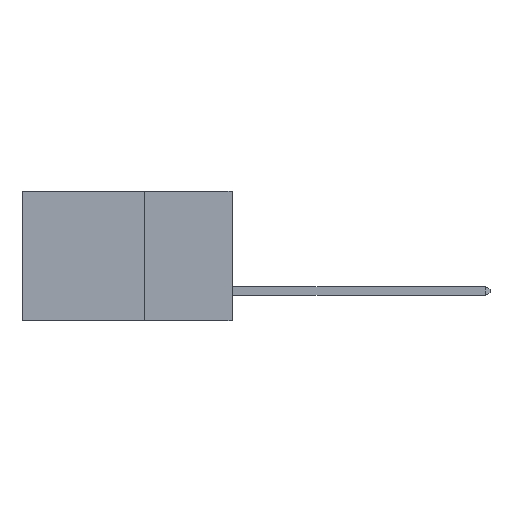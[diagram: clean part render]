
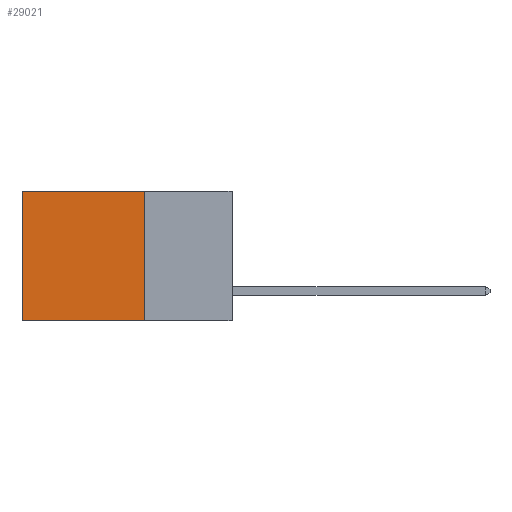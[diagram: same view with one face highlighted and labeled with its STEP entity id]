
A CAD part, left-side view. The second image highlights one B-rep face of the part: STEP entity #29021.
In plain terms, the highlighted planar face has unit normal (-1, 0, 0).
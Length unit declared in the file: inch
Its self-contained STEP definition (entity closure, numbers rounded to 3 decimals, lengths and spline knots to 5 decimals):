
#391 = EDGE_LOOP ( 'NONE', ( #3267, #21433, #400, #19295 ) ) ;
#400 = ORIENTED_EDGE ( 'NONE', *, *, #24322, .F. ) ;
#2300 = VECTOR ( 'NONE', #9918, 39.37008 ) ;
#2621 = DIRECTION ( 'NONE',  ( 0., 0., -1. ) ) ;
#3267 = ORIENTED_EDGE ( 'NONE', *, *, #25657, .T. ) ;
#4385 = CARTESIAN_POINT ( 'NONE',  ( 0.2875, 0.6, 0. ) ) ;
#4949 = CARTESIAN_POINT ( 'NONE',  ( 0.2875, 0.25, 0. ) ) ;
#5267 = LINE ( 'NONE', #7214, #10579 ) ;
#7214 = CARTESIAN_POINT ( 'NONE',  ( 0.2875, 0.25, 0. ) ) ;
#7243 = DIRECTION ( 'NONE',  ( 0., 0., -1. ) ) ;
#7645 = CARTESIAN_POINT ( 'NONE',  ( 0.2875, 0.6, 0. ) ) ;
#8016 = VECTOR ( 'NONE', #23981, 39.37008 ) ;
#9410 = PLANE ( 'NONE',  #14058 ) ;
#9580 = CARTESIAN_POINT ( 'NONE',  ( 0.2875, 0.25, -0.37 ) ) ;
#9918 = DIRECTION ( 'NONE',  ( 0., 0., -1. ) ) ;
#10579 = VECTOR ( 'NONE', #2621, 39.37008 ) ;
#11506 = CARTESIAN_POINT ( 'NONE',  ( 0.2875, 0.6, -0.37 ) ) ;
#11764 = VECTOR ( 'NONE', #16145, 39.37008 ) ;
#13355 = LINE ( 'NONE', #21733, #8016 ) ;
#13739 = VERTEX_POINT ( 'NONE', #9580 ) ;
#14058 = AXIS2_PLACEMENT_3D ( 'NONE', #4949, #20661, #7243 ) ;
#14249 = FACE_OUTER_BOUND ( 'NONE', #391, .T. ) ;
#16145 = DIRECTION ( 'NONE',  ( 0., 1., 0. ) ) ;
#17350 = VERTEX_POINT ( 'NONE', #11506 ) ;
#17398 = EDGE_CURVE ( 'NONE', #13739, #17350, #17724, .T. ) ;
#17724 = LINE ( 'NONE', #22824, #11764 ) ;
#19295 = ORIENTED_EDGE ( 'NONE', *, *, #25839, .T. ) ;
#19588 = LINE ( 'NONE', #7645, #2300 ) ;
#19792 = VERTEX_POINT ( 'NONE', #4385 ) ;
#20661 = DIRECTION ( 'NONE',  ( 1., 0., 0. ) ) ;
#21433 = ORIENTED_EDGE ( 'NONE', *, *, #17398, .F. ) ;
#21733 = CARTESIAN_POINT ( 'NONE',  ( 0.2875, 0.25, 0. ) ) ;
#22824 = CARTESIAN_POINT ( 'NONE',  ( 0.2875, 0.25, -0.37 ) ) ;
#23105 = CARTESIAN_POINT ( 'NONE',  ( 0.2875, 0.25, 0. ) ) ;
#23981 = DIRECTION ( 'NONE',  ( 0., 1., 0. ) ) ;
#24322 = EDGE_CURVE ( 'NONE', #25596, #13739, #5267, .T. ) ;
#25596 = VERTEX_POINT ( 'NONE', #23105 ) ;
#25657 = EDGE_CURVE ( 'NONE', #19792, #17350, #19588, .T. ) ;
#25839 = EDGE_CURVE ( 'NONE', #25596, #19792, #13355, .T. ) ;
#29021 = ADVANCED_FACE ( 'NONE', ( #14249 ), #9410, .F. ) ;
